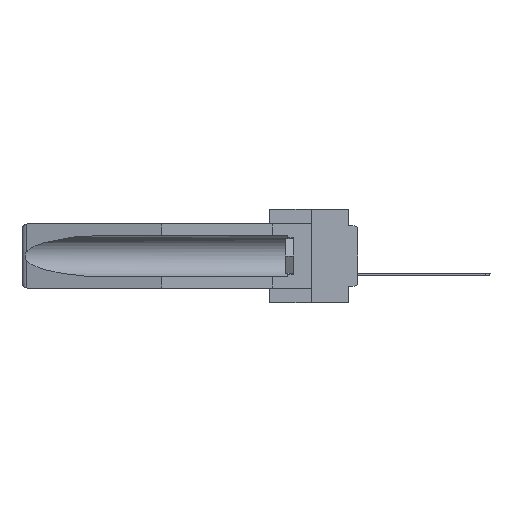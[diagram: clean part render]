
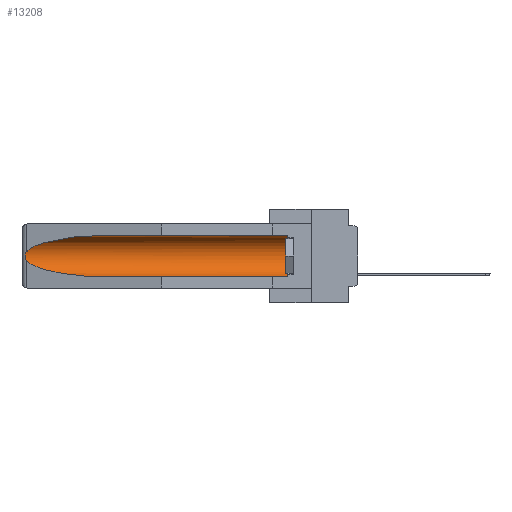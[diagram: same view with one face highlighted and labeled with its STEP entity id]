
A CAD part, left-side view. The second image highlights one B-rep face of the part: STEP entity #13208.
In plain terms, the highlighted cylindrical face has radius 2.857 mm (diameter 5.715 mm), a partial arc.
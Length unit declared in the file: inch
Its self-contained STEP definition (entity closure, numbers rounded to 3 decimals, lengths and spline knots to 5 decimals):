
#695 = B_SPLINE_CURVE_WITH_KNOTS ( 'NONE', 3,
 ( #19446, #3695, #1623, #20032, #12230, #14955, #20825, #19369, #18350, #28924 ),
 .UNSPECIFIED., .F., .F.,
 ( 4, 2, 2, 2, 4 ),
 ( 0., 0.00029, 0.00058, 0.00087, 0.00117 ),
 .UNSPECIFIED. ) ;
#1623 = CARTESIAN_POINT ( 'NONE',  ( 0.26654, 1.53092, -0.15636 ) ) ;
#2445 = FACE_OUTER_BOUND ( 'NONE', #27296, .T. ) ;
#3695 = CARTESIAN_POINT ( 'NONE',  ( 0.26597, 1.52961, -0.15275 ) ) ;
#4070 = CARTESIAN_POINT ( 'NONE',  ( 0.26537, 1.52718, -0.14972 ) ) ;
#4125 = ORIENTED_EDGE ( 'NONE', *, *, #15752, .T. ) ;
#4763 = VERTEX_POINT ( 'NONE', #18004 ) ;
#6513 = CARTESIAN_POINT ( 'NONE',  ( 0.155, 1.07973, -0.059 ) ) ;
#7586 = VERTEX_POINT ( 'NONE', #30485 ) ;
#7719 = CARTESIAN_POINT ( 'NONE',  ( 0.155, 1.07973, -0.059 ) ) ;
#8033 = VECTOR ( 'NONE', #29139, 39.37008 ) ;
#8908 = ORIENTED_EDGE ( 'NONE', *, *, #17341, .T. ) ;
#10445 = VERTEX_POINT ( 'NONE', #14989 ) ;
#11205 = CARTESIAN_POINT ( 'NONE',  ( 0.26537, 1.52718, -0.19328 ) ) ;
#11269 = CARTESIAN_POINT ( 'NONE',  ( 0.26537, 1.52718, -0.19328 ) ) ;
#11771 = VERTEX_POINT ( 'NONE', #4070 ) ;
#12066 = CARTESIAN_POINT ( 'NONE',  ( 0.155, -0.30754, -0.1715 ) ) ;
#12230 = CARTESIAN_POINT ( 'NONE',  ( 0.2675, 1.53308, -0.16763 ) ) ;
#13208 = ADVANCED_FACE ( 'NONE', ( #2445 ), #24655, .F. ) ;
#13606 = CARTESIAN_POINT ( 'NONE',  ( 0.155, -0.30754, -0.284 ) ) ;
#14304 = CARTESIAN_POINT ( 'NONE',  ( 0.155, 1.07973, -0.284 ) ) ;
#14641 = VERTEX_POINT ( 'NONE', #11269 ) ;
#14907 = DIRECTION ( 'NONE',  ( 0., 0., 1. ) ) ;
#14955 = CARTESIAN_POINT ( 'NONE',  ( 0.2675, 1.53308, -0.17534 ) ) ;
#14989 = CARTESIAN_POINT ( 'NONE',  ( 0.155, 0.126, -0.284 ) ) ;
#15657 = ORIENTED_EDGE ( 'NONE', *, *, #18237, .T. ) ;
#15752 = EDGE_CURVE ( 'NONE', #14641, #7586, #18676, .T. ) ;
#15768 = DIRECTION ( 'NONE',  ( 0., -1., 0. ) ) ;
#16376 = EDGE_CURVE ( 'NONE', #10445, #4763, #30494, .T. ) ;
#16969 = CARTESIAN_POINT ( 'NONE',  ( 0.26537, 1.52718, -0.14972 ) ) ;
#17341 = EDGE_CURVE ( 'NONE', #11771, #14641, #695, .T. ) ;
#18004 = CARTESIAN_POINT ( 'NONE',  ( 0.155, 0.126, -0.059 ) ) ;
#18237 = EDGE_CURVE ( 'NONE', #27940, #11771, #25195, .T. ) ;
#18350 = CARTESIAN_POINT ( 'NONE',  ( 0.26597, 1.5296, -0.19026 ) ) ;
#18676 =( BOUNDED_CURVE ( )  B_SPLINE_CURVE ( 3, ( #11205, #30858, #32934, #14304 ),
 .UNSPECIFIED., .F., .F. ) 
 B_SPLINE_CURVE_WITH_KNOTS ( ( 4, 4 ),
 ( 0.1948, 1.5708 ),
 .UNSPECIFIED. ) 
 CURVE ( )  GEOMETRIC_REPRESENTATION_ITEM ( )  RATIONAL_B_SPLINE_CURVE ( ( 1., 0.848, 0.848, 1. ) ) 
 REPRESENTATION_ITEM ( '' )  );
#19168 = AXIS2_PLACEMENT_3D ( 'NONE', #12066, #20093, #14907 ) ;
#19204 = EDGE_CURVE ( 'NONE', #10445, #7586, #26524, .T. ) ;
#19369 = CARTESIAN_POINT ( 'NONE',  ( 0.26655, 1.53094, -0.18657 ) ) ;
#19446 = CARTESIAN_POINT ( 'NONE',  ( 0.26537, 1.52718, -0.14972 ) ) ;
#19484 = ORIENTED_EDGE ( 'NONE', *, *, #19204, .F. ) ;
#19504 = CARTESIAN_POINT ( 'NONE',  ( 0.25451, 1.48313, -0.09465 ) ) ;
#20032 = CARTESIAN_POINT ( 'NONE',  ( 0.2673, 1.5327, -0.16383 ) ) ;
#20093 = DIRECTION ( 'NONE',  ( 0., 1., 0. ) ) ;
#20825 = CARTESIAN_POINT ( 'NONE',  ( 0.2673, 1.53269, -0.17917 ) ) ;
#20999 = AXIS2_PLACEMENT_3D ( 'NONE', #32452, #15768, #21070 ) ;
#21070 = DIRECTION ( 'NONE',  ( 0., 0., 1. ) ) ;
#23757 = EDGE_CURVE ( 'NONE', #4763, #27940, #26778, .T. ) ;
#24655 = CYLINDRICAL_SURFACE ( 'NONE', #19168, 0.1125 ) ;
#24779 = VECTOR ( 'NONE', #29226, 39.37008 ) ;
#25195 =( BOUNDED_CURVE ( )  B_SPLINE_CURVE ( 3, ( #6513, #30061, #19504, #16969 ),
 .UNSPECIFIED., .F., .F. ) 
 B_SPLINE_CURVE_WITH_KNOTS ( ( 4, 4 ),
 ( 4.71239, 6.08839 ),
 .UNSPECIFIED. ) 
 CURVE ( )  GEOMETRIC_REPRESENTATION_ITEM ( )  RATIONAL_B_SPLINE_CURVE ( ( 1., 0.848, 0.848, 1. ) ) 
 REPRESENTATION_ITEM ( '' )  );
#26524 = LINE ( 'NONE', #13606, #8033 ) ;
#26778 = LINE ( 'NONE', #27029, #24779 ) ;
#27029 = CARTESIAN_POINT ( 'NONE',  ( 0.155, -0.30754, -0.059 ) ) ;
#27296 = EDGE_LOOP ( 'NONE', ( #15657, #8908, #4125, #19484, #33749, #31480 ) ) ;
#27940 = VERTEX_POINT ( 'NONE', #7719 ) ;
#28924 = CARTESIAN_POINT ( 'NONE',  ( 0.26537, 1.52718, -0.19328 ) ) ;
#29139 = DIRECTION ( 'NONE',  ( 0., 1., 0. ) ) ;
#29226 = DIRECTION ( 'NONE',  ( 0., 1., 0. ) ) ;
#30061 = CARTESIAN_POINT ( 'NONE',  ( 0.21114, 1.30732, -0.059 ) ) ;
#30485 = CARTESIAN_POINT ( 'NONE',  ( 0.155, 1.07973, -0.284 ) ) ;
#30494 = CIRCLE ( 'NONE', #20999, 0.1125 ) ;
#30858 = CARTESIAN_POINT ( 'NONE',  ( 0.25451, 1.48313, -0.24835 ) ) ;
#31480 = ORIENTED_EDGE ( 'NONE', *, *, #23757, .T. ) ;
#32452 = CARTESIAN_POINT ( 'NONE',  ( 0.155, 0.126, -0.1715 ) ) ;
#32934 = CARTESIAN_POINT ( 'NONE',  ( 0.21114, 1.30732, -0.284 ) ) ;
#33749 = ORIENTED_EDGE ( 'NONE', *, *, #16376, .T. ) ;
